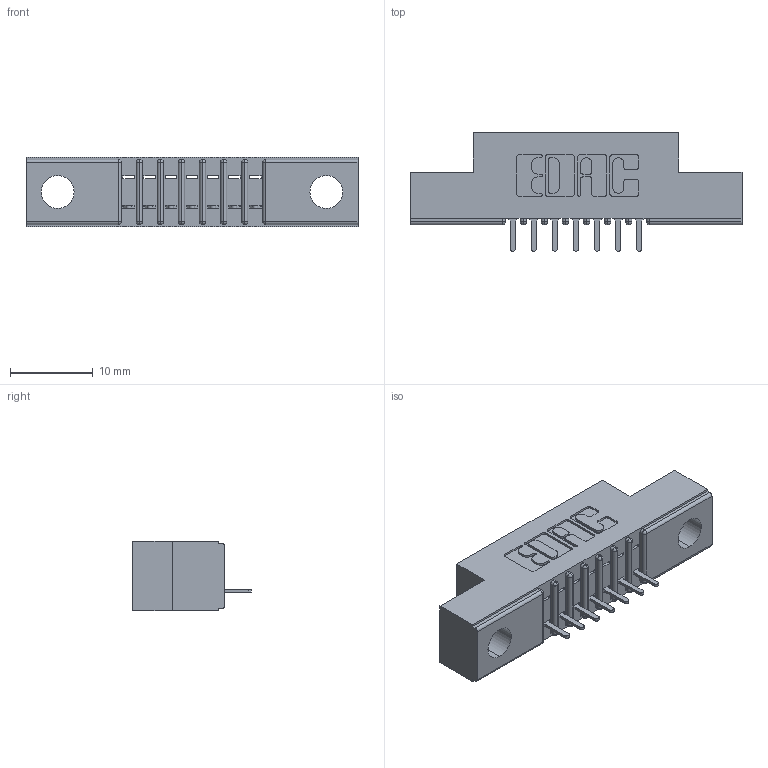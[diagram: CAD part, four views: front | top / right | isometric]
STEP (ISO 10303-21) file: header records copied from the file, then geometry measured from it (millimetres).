
FILE_DESCRIPTION (( 'STEP AP203' ), '1' );
FILE_NAME ('391-007-520-104.STEP', '2018-08-08T15:25:01', ( '' ), ( '' ), 'SwSTEP 2.0', 'SolidWorks 2016', '' );
FILE_SCHEMA (( 'CONFIG_CONTROL_DESIGN' ));
Length unit declared in the file: inch
Products named in the file (3): 391-007-520-104; 341 Part_.156 (3.96) Dia Mounting Holes; 341-292-001_341-292-120
Assembly tree (8 placements, depth 2):
  391-007-520-104
    341 Part_.156 (3.96) Dia Mounting Holes
    341-292-001_341-292-120  x7
Bounding box: 40.01 x 14.27 x 8.38 mm (x, y, z)
Volume: 2162.7 mm3; surface area: 3160.1 mm2
Topology: 8 solids, 8 shells, 704 faces, 2011 edges, 1294 vertices
Faces by surface type: plane 439, cylinder 237, sphere 16, torus 12
Entity records: 13328 total; most frequent: CARTESIAN_POINT 2252, ORIENTED_EDGE 2238, DIRECTION 2195, EDGE_CURVE 1119, LINE 873, VECTOR 873, VERTEX_POINT 718, AXIS2_PLACEMENT_3D 661
